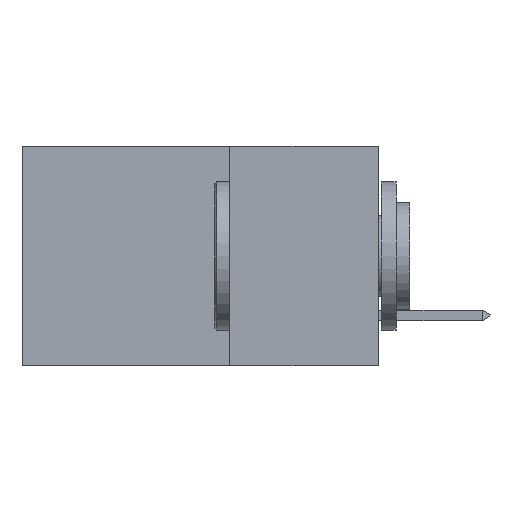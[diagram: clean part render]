
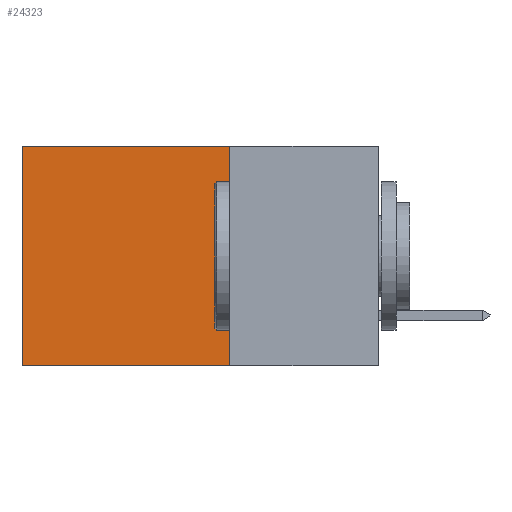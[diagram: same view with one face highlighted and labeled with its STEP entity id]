
A CAD part, left-side view. The second image highlights one B-rep face of the part: STEP entity #24323.
In plain terms, the highlighted planar face has unit normal (-1, 0, 0).
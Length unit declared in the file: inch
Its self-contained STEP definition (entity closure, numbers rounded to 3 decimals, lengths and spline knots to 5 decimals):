
#131 = CARTESIAN_POINT ( 'NONE',  ( 0.2615, 0.25, 0. ) ) ;
#259 = DIRECTION ( 'NONE',  ( 0., 1., 0. ) ) ;
#974 = VECTOR ( 'NONE', #259, 39.37008 ) ;
#2100 = DIRECTION ( 'NONE',  ( 0., 0., -1. ) ) ;
#5436 = EDGE_CURVE ( 'NONE', #15289, #8617, #15688, .T. ) ;
#6474 = VECTOR ( 'NONE', #11310, 39.37008 ) ;
#6665 = VERTEX_POINT ( 'NONE', #8901 ) ;
#7190 = FACE_OUTER_BOUND ( 'NONE', #17198, .T. ) ;
#7320 = EDGE_CURVE ( 'NONE', #8617, #6665, #12558, .T. ) ;
#7419 = VECTOR ( 'NONE', #11907, 39.37008 ) ;
#8043 = CARTESIAN_POINT ( 'NONE',  ( 0.2615, 0.25, -0.37 ) ) ;
#8126 = DIRECTION ( 'NONE',  ( 0., 1., 0. ) ) ;
#8503 = CARTESIAN_POINT ( 'NONE',  ( 0.2615, 0.25, -0.37 ) ) ;
#8617 = VERTEX_POINT ( 'NONE', #12971 ) ;
#8901 = CARTESIAN_POINT ( 'NONE',  ( 0.2615, 0.6, -0.37 ) ) ;
#9390 = CARTESIAN_POINT ( 'NONE',  ( 0.2615, 0.25, -0.37 ) ) ;
#9443 = ORIENTED_EDGE ( 'NONE', *, *, #19838, .F. ) ;
#10163 = LINE ( 'NONE', #8043, #19794 ) ;
#10401 = AXIS2_PLACEMENT_3D ( 'NONE', #17317, #13633, #2100 ) ;
#11310 = DIRECTION ( 'NONE',  ( 0., 0., -1. ) ) ;
#11637 = PLANE ( 'NONE',  #10401 ) ;
#11870 = CARTESIAN_POINT ( 'NONE',  ( 0.2615, 0.6, -0.37 ) ) ;
#11907 = DIRECTION ( 'NONE',  ( 0., 0., -1. ) ) ;
#12558 = LINE ( 'NONE', #11870, #7419 ) ;
#12971 = CARTESIAN_POINT ( 'NONE',  ( 0.2615, 0.6, 0. ) ) ;
#13333 = ORIENTED_EDGE ( 'NONE', *, *, #5436, .T. ) ;
#13479 = VERTEX_POINT ( 'NONE', #8503 ) ;
#13633 = DIRECTION ( 'NONE',  ( 1., 0., 0. ) ) ;
#15289 = VERTEX_POINT ( 'NONE', #19677 ) ;
#15688 = LINE ( 'NONE', #131, #974 ) ;
#16877 = ORIENTED_EDGE ( 'NONE', *, *, #18425, .F. ) ;
#17198 = EDGE_LOOP ( 'NONE', ( #19820, #16877, #9443, #13333 ) ) ;
#17317 = CARTESIAN_POINT ( 'NONE',  ( 0.2615, 0.25, -0.37 ) ) ;
#18425 = EDGE_CURVE ( 'NONE', #13479, #6665, #10163, .T. ) ;
#19677 = CARTESIAN_POINT ( 'NONE',  ( 0.2615, 0.25, 0. ) ) ;
#19794 = VECTOR ( 'NONE', #8126, 39.37008 ) ;
#19820 = ORIENTED_EDGE ( 'NONE', *, *, #7320, .T. ) ;
#19838 = EDGE_CURVE ( 'NONE', #15289, #13479, #21728, .T. ) ;
#21728 = LINE ( 'NONE', #9390, #6474 ) ;
#24323 = ADVANCED_FACE ( 'NONE', ( #7190 ), #11637, .F. ) ;
